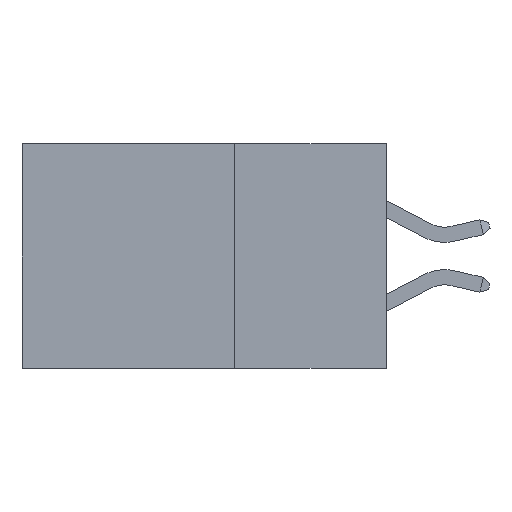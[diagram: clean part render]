
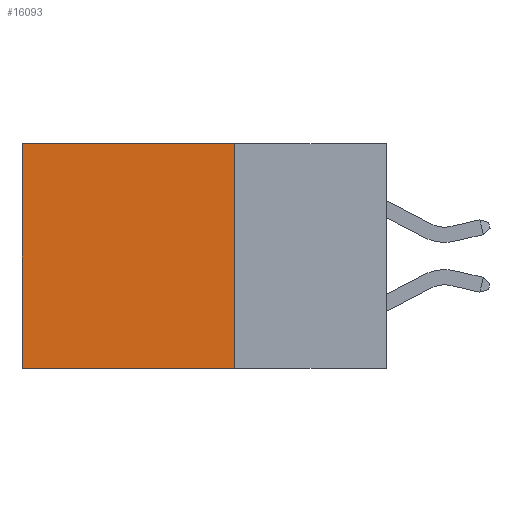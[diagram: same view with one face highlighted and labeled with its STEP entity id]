
A CAD part, left-side view. The second image highlights one B-rep face of the part: STEP entity #16093.
In plain terms, the highlighted planar face has unit normal (-1, 0, 0).
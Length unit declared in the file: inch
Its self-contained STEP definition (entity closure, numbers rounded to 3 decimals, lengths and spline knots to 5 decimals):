
#479 = DIRECTION ( 'NONE',  ( 0., 0., -1. ) ) ;
#3217 = LINE ( 'NONE', #12208, #9853 ) ;
#3307 = DIRECTION ( 'NONE',  ( 0., 0., -1. ) ) ;
#3819 = EDGE_LOOP ( 'NONE', ( #16958, #11113, #11107, #16393 ) ) ;
#4451 = LINE ( 'NONE', #17715, #6112 ) ;
#5103 = FACE_OUTER_BOUND ( 'NONE', #3819, .T. ) ;
#5264 = VERTEX_POINT ( 'NONE', #9023 ) ;
#5670 = VERTEX_POINT ( 'NONE', #13081 ) ;
#6010 = LINE ( 'NONE', #9231, #10154 ) ;
#6112 = VECTOR ( 'NONE', #16103, 39.37008 ) ;
#6427 = DIRECTION ( 'NONE',  ( 0., 0., -1. ) ) ;
#9023 = CARTESIAN_POINT ( 'NONE',  ( 0.2615, 0.6, 0. ) ) ;
#9231 = CARTESIAN_POINT ( 'NONE',  ( 0.2615, 0.25, 0. ) ) ;
#9715 = CARTESIAN_POINT ( 'NONE',  ( 0.2615, 0.25, -0.37 ) ) ;
#9853 = VECTOR ( 'NONE', #479, 39.37008 ) ;
#9926 = EDGE_CURVE ( 'NONE', #5670, #5264, #6010, .T. ) ;
#10154 = VECTOR ( 'NONE', #10562, 39.37008 ) ;
#10161 = CARTESIAN_POINT ( 'NONE',  ( 0.2615, 0.6, -0.37 ) ) ;
#10249 = EDGE_CURVE ( 'NONE', #5670, #15427, #11395, .T. ) ;
#10286 = EDGE_CURVE ( 'NONE', #5264, #12917, #3217, .T. ) ;
#10516 = CARTESIAN_POINT ( 'NONE',  ( 0.2615, 0.25, -0.37 ) ) ;
#10562 = DIRECTION ( 'NONE',  ( 0., 1., 0. ) ) ;
#10605 = CARTESIAN_POINT ( 'NONE',  ( 0.2615, 0.25, -0.37 ) ) ;
#10972 = DIRECTION ( 'NONE',  ( 1., 0., 0. ) ) ;
#11107 = ORIENTED_EDGE ( 'NONE', *, *, #10249, .F. ) ;
#11113 = ORIENTED_EDGE ( 'NONE', *, *, #18562, .F. ) ;
#11395 = LINE ( 'NONE', #10516, #15307 ) ;
#12208 = CARTESIAN_POINT ( 'NONE',  ( 0.2615, 0.6, -0.37 ) ) ;
#12917 = VERTEX_POINT ( 'NONE', #10161 ) ;
#13058 = AXIS2_PLACEMENT_3D ( 'NONE', #10605, #10972, #6427 ) ;
#13081 = CARTESIAN_POINT ( 'NONE',  ( 0.2615, 0.25, 0. ) ) ;
#15307 = VECTOR ( 'NONE', #3307, 39.37008 ) ;
#15427 = VERTEX_POINT ( 'NONE', #9715 ) ;
#16093 = ADVANCED_FACE ( 'NONE', ( #5103 ), #16377, .F. ) ;
#16103 = DIRECTION ( 'NONE',  ( 0., 1., 0. ) ) ;
#16377 = PLANE ( 'NONE',  #13058 ) ;
#16393 = ORIENTED_EDGE ( 'NONE', *, *, #9926, .T. ) ;
#16958 = ORIENTED_EDGE ( 'NONE', *, *, #10286, .T. ) ;
#17715 = CARTESIAN_POINT ( 'NONE',  ( 0.2615, 0.25, -0.37 ) ) ;
#18562 = EDGE_CURVE ( 'NONE', #15427, #12917, #4451, .T. ) ;
